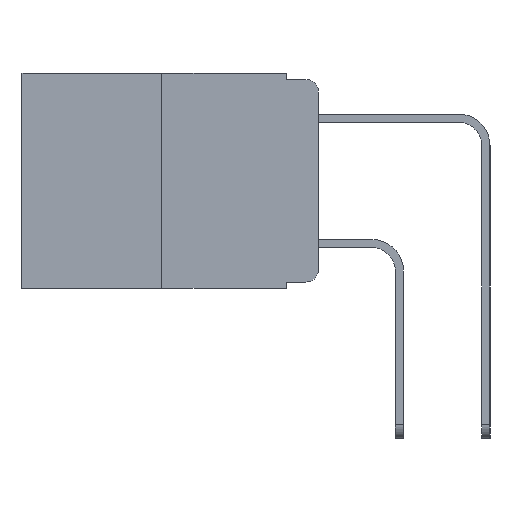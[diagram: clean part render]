
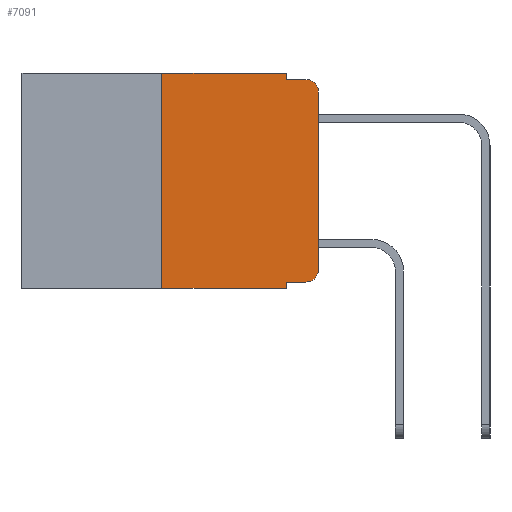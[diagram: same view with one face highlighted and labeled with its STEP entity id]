
A CAD part, left-side view. The second image highlights one B-rep face of the part: STEP entity #7091.
In plain terms, the highlighted planar face has unit normal (-1, 0, 0).
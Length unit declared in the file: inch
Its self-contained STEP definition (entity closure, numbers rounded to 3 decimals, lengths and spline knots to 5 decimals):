
#83 = CARTESIAN_POINT ( 'NONE',  ( 0., 0.02, -0.01 ) ) ;
#113 = VERTEX_POINT ( 'NONE', #10764 ) ;
#548 = DIRECTION ( 'NONE',  ( 0., 0., -1. ) ) ;
#748 = VECTOR ( 'NONE', #5823, 39.37008 ) ;
#819 = VECTOR ( 'NONE', #3839, 39.37008 ) ;
#909 = DIRECTION ( 'NONE',  ( 0., 0., -1. ) ) ;
#1028 = EDGE_CURVE ( 'NONE', #10605, #5909, #9381, .T. ) ;
#1352 = DIRECTION ( 'NONE',  ( 0., 0., 1. ) ) ;
#1405 = AXIS2_PLACEMENT_3D ( 'NONE', #8328, #1964, #9334 ) ;
#1707 = EDGE_CURVE ( 'NONE', #10605, #113, #13411, .T. ) ;
#1964 = DIRECTION ( 'NONE',  ( -1., 0., 0. ) ) ;
#1980 = VECTOR ( 'NONE', #1352, 39.37008 ) ;
#2209 = ORIENTED_EDGE ( 'NONE', *, *, #12996, .T. ) ;
#2392 = CARTESIAN_POINT ( 'NONE',  ( 0., 0., -0.313 ) ) ;
#2394 = CIRCLE ( 'NONE', #1405, 0.02 ) ;
#2649 = AXIS2_PLACEMENT_3D ( 'NONE', #13083, #7052, #548 ) ;
#2814 = PLANE ( 'NONE',  #7075 ) ;
#2953 = CARTESIAN_POINT ( 'NONE',  ( 0., 0., 0. ) ) ;
#3220 = CARTESIAN_POINT ( 'NONE',  ( 0., 0.051, -0.333 ) ) ;
#3493 = EDGE_CURVE ( 'NONE', #9106, #5363, #2394, .T. ) ;
#3618 = CARTESIAN_POINT ( 'NONE',  ( 0., 0., -0.03 ) ) ;
#3839 = DIRECTION ( 'NONE',  ( 0., -1., 0. ) ) ;
#3966 = CARTESIAN_POINT ( 'NONE',  ( 0., 0.051, -0.01 ) ) ;
#3973 = ORIENTED_EDGE ( 'NONE', *, *, #1028, .F. ) ;
#4047 = CARTESIAN_POINT ( 'NONE',  ( 0., 0.051, -0.01 ) ) ;
#4234 = CARTESIAN_POINT ( 'NONE',  ( 0., 0.051, 0. ) ) ;
#4347 = VECTOR ( 'NONE', #11088, 39.37008 ) ;
#4613 = ORIENTED_EDGE ( 'NONE', *, *, #13578, .F. ) ;
#4717 = FACE_OUTER_BOUND ( 'NONE', #8054, .T. ) ;
#4771 = CARTESIAN_POINT ( 'NONE',  ( 0., 0.473, -0.343 ) ) ;
#5023 = CARTESIAN_POINT ( 'NONE',  ( 0., 0.473, 0. ) ) ;
#5363 = VERTEX_POINT ( 'NONE', #83 ) ;
#5405 = CARTESIAN_POINT ( 'NONE',  ( 0., 0.051, -0.333 ) ) ;
#5669 = VECTOR ( 'NONE', #12455, 39.37008 ) ;
#5670 = CARTESIAN_POINT ( 'NONE',  ( 0., 0.25, 0. ) ) ;
#5823 = DIRECTION ( 'NONE',  ( 0., -1., 0. ) ) ;
#5909 = VERTEX_POINT ( 'NONE', #8434 ) ;
#6086 = DIRECTION ( 'NONE',  ( 1., 0., 0. ) ) ;
#6482 = VERTEX_POINT ( 'NONE', #9300 ) ;
#6516 = ORIENTED_EDGE ( 'NONE', *, *, #8712, .F. ) ;
#6567 = CIRCLE ( 'NONE', #2649, 0.02 ) ;
#6595 = LINE ( 'NONE', #12987, #819 ) ;
#6781 = LINE ( 'NONE', #3966, #4347 ) ;
#6839 = ORIENTED_EDGE ( 'NONE', *, *, #7335, .F. ) ;
#6957 = VECTOR ( 'NONE', #8216, 39.37008 ) ;
#7052 = DIRECTION ( 'NONE',  ( -1., 0., 0. ) ) ;
#7075 = AXIS2_PLACEMENT_3D ( 'NONE', #5023, #6086, #13126 ) ;
#7091 = ADVANCED_FACE ( 'NONE', ( #4717 ), #2814, .F. ) ;
#7164 = VERTEX_POINT ( 'NONE', #4047 ) ;
#7335 = EDGE_CURVE ( 'NONE', #6482, #7164, #12962, .T. ) ;
#7550 = ORIENTED_EDGE ( 'NONE', *, *, #1707, .T. ) ;
#8020 = EDGE_CURVE ( 'NONE', #10774, #9106, #12299, .T. ) ;
#8054 = EDGE_LOOP ( 'NONE', ( #9037, #11193, #6516, #6839, #10857, #4613, #2209, #3973, #7550, #8765 ) ) ;
#8216 = DIRECTION ( 'NONE',  ( 0., 0., 1. ) ) ;
#8224 = VERTEX_POINT ( 'NONE', #13488 ) ;
#8328 = CARTESIAN_POINT ( 'NONE',  ( 0., 0.02, -0.03 ) ) ;
#8434 = CARTESIAN_POINT ( 'NONE',  ( 0., 0.051, -0.343 ) ) ;
#8712 = EDGE_CURVE ( 'NONE', #7164, #5363, #6781, .T. ) ;
#8765 = ORIENTED_EDGE ( 'NONE', *, *, #11014, .T. ) ;
#9037 = ORIENTED_EDGE ( 'NONE', *, *, #8020, .T. ) ;
#9058 = VECTOR ( 'NONE', #10324, 39.37008 ) ;
#9106 = VERTEX_POINT ( 'NONE', #3618 ) ;
#9251 = LINE ( 'NONE', #4771, #748 ) ;
#9300 = CARTESIAN_POINT ( 'NONE',  ( 0., 0.051, 0. ) ) ;
#9319 = CARTESIAN_POINT ( 'NONE',  ( 0., 0.051, 0. ) ) ;
#9334 = DIRECTION ( 'NONE',  ( 0., 0., -1. ) ) ;
#9381 = LINE ( 'NONE', #9319, #9058 ) ;
#9713 = EDGE_CURVE ( 'NONE', #8224, #6482, #6595, .T. ) ;
#10098 = VERTEX_POINT ( 'NONE', #11623 ) ;
#10307 = VECTOR ( 'NONE', #909, 39.37008 ) ;
#10324 = DIRECTION ( 'NONE',  ( 0., 0., -1. ) ) ;
#10605 = VERTEX_POINT ( 'NONE', #5405 ) ;
#10764 = CARTESIAN_POINT ( 'NONE',  ( 0., 0.02, -0.333 ) ) ;
#10774 = VERTEX_POINT ( 'NONE', #2392 ) ;
#10857 = ORIENTED_EDGE ( 'NONE', *, *, #9713, .F. ) ;
#11014 = EDGE_CURVE ( 'NONE', #113, #10774, #6567, .T. ) ;
#11088 = DIRECTION ( 'NONE',  ( 0., -1., 0. ) ) ;
#11193 = ORIENTED_EDGE ( 'NONE', *, *, #3493, .T. ) ;
#11623 = CARTESIAN_POINT ( 'NONE',  ( 0., 0.25, -0.343 ) ) ;
#12299 = LINE ( 'NONE', #2953, #6957 ) ;
#12455 = DIRECTION ( 'NONE',  ( 0., -1., 0. ) ) ;
#12962 = LINE ( 'NONE', #4234, #10307 ) ;
#12982 = LINE ( 'NONE', #5670, #1980 ) ;
#12987 = CARTESIAN_POINT ( 'NONE',  ( 0., 0.473, 0. ) ) ;
#12996 = EDGE_CURVE ( 'NONE', #10098, #5909, #9251, .T. ) ;
#13083 = CARTESIAN_POINT ( 'NONE',  ( 0., 0.02, -0.313 ) ) ;
#13126 = DIRECTION ( 'NONE',  ( 0., 0., -1. ) ) ;
#13411 = LINE ( 'NONE', #3220, #5669 ) ;
#13488 = CARTESIAN_POINT ( 'NONE',  ( 0., 0.25, 0. ) ) ;
#13578 = EDGE_CURVE ( 'NONE', #10098, #8224, #12982, .T. ) ;
